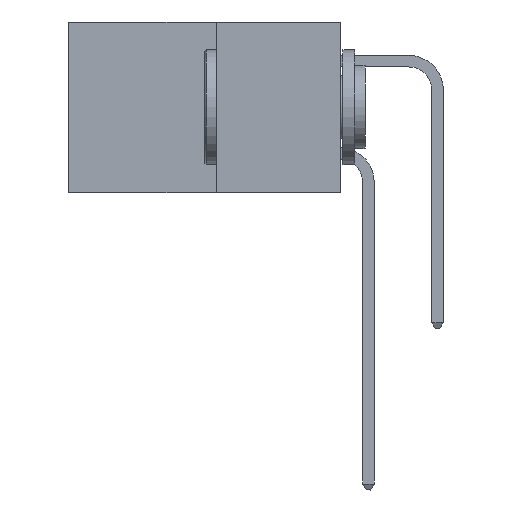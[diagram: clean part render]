
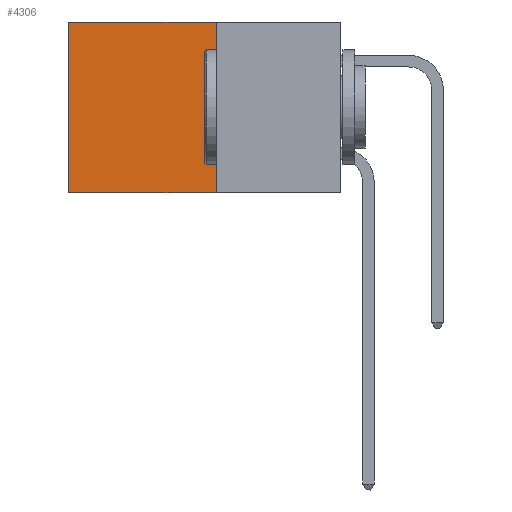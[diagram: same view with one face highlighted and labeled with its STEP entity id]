
A CAD part, left-side view. The second image highlights one B-rep face of the part: STEP entity #4306.
In plain terms, the highlighted planar face has unit normal (-1, 0, 0).
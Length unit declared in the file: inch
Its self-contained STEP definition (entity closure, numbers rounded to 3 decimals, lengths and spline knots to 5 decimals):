
#726 = CARTESIAN_POINT ( 'NONE',  ( 0.277, 0.27, 0. ) ) ;
#907 = CARTESIAN_POINT ( 'NONE',  ( 0.277, 0.27, -0.37 ) ) ;
#1621 = EDGE_CURVE ( 'NONE', #27426, #2841, #13937, .T. ) ;
#2651 = VERTEX_POINT ( 'NONE', #18108 ) ;
#2778 = LINE ( 'NONE', #907, #14039 ) ;
#2841 = VERTEX_POINT ( 'NONE', #24920 ) ;
#3129 = DIRECTION ( 'NONE',  ( 0., 1., 0. ) ) ;
#4264 = CARTESIAN_POINT ( 'NONE',  ( 0.277, 0.59, -0.37 ) ) ;
#4306 = ADVANCED_FACE ( 'NONE', ( #15895 ), #20793, .F. ) ;
#5614 = LINE ( 'NONE', #4264, #11643 ) ;
#7974 = VECTOR ( 'NONE', #10528, 39.37008 ) ;
#8885 = EDGE_CURVE ( 'NONE', #27426, #16696, #11037, .T. ) ;
#10528 = DIRECTION ( 'NONE',  ( 0., 1., 0. ) ) ;
#10722 = EDGE_CURVE ( 'NONE', #2841, #2651, #5614, .T. ) ;
#10831 = DIRECTION ( 'NONE',  ( 0., 0., -1. ) ) ;
#11037 = LINE ( 'NONE', #28577, #27357 ) ;
#11643 = VECTOR ( 'NONE', #26540, 39.37008 ) ;
#13937 = LINE ( 'NONE', #726, #7974 ) ;
#14039 = VECTOR ( 'NONE', #3129, 39.37008 ) ;
#14576 = AXIS2_PLACEMENT_3D ( 'NONE', #20770, #20763, #20740 ) ;
#15693 = CARTESIAN_POINT ( 'NONE',  ( 0.277, 0.27, 0. ) ) ;
#15895 = FACE_OUTER_BOUND ( 'NONE', #23547, .T. ) ;
#16696 = VERTEX_POINT ( 'NONE', #23871 ) ;
#17244 = ORIENTED_EDGE ( 'NONE', *, *, #10722, .T. ) ;
#17872 = EDGE_CURVE ( 'NONE', #16696, #2651, #2778, .T. ) ;
#18108 = CARTESIAN_POINT ( 'NONE',  ( 0.277, 0.59, -0.37 ) ) ;
#20740 = DIRECTION ( 'NONE',  ( 0., 0., -1. ) ) ;
#20763 = DIRECTION ( 'NONE',  ( 1., 0., 0. ) ) ;
#20770 = CARTESIAN_POINT ( 'NONE',  ( 0.277, 0.27, -0.37 ) ) ;
#20793 = PLANE ( 'NONE',  #14576 ) ;
#21125 = ORIENTED_EDGE ( 'NONE', *, *, #8885, .F. ) ;
#21455 = ORIENTED_EDGE ( 'NONE', *, *, #17872, .F. ) ;
#22557 = ORIENTED_EDGE ( 'NONE', *, *, #1621, .T. ) ;
#23547 = EDGE_LOOP ( 'NONE', ( #17244, #21455, #21125, #22557 ) ) ;
#23871 = CARTESIAN_POINT ( 'NONE',  ( 0.277, 0.27, -0.37 ) ) ;
#24920 = CARTESIAN_POINT ( 'NONE',  ( 0.277, 0.59, 0. ) ) ;
#26540 = DIRECTION ( 'NONE',  ( 0., 0., -1. ) ) ;
#27357 = VECTOR ( 'NONE', #10831, 39.37008 ) ;
#27426 = VERTEX_POINT ( 'NONE', #15693 ) ;
#28577 = CARTESIAN_POINT ( 'NONE',  ( 0.277, 0.27, -0.37 ) ) ;
